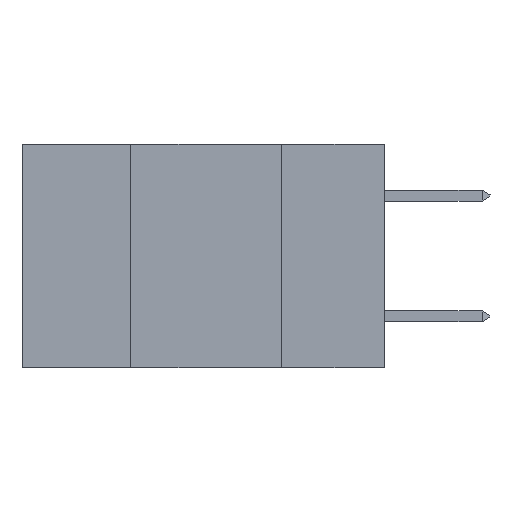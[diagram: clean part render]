
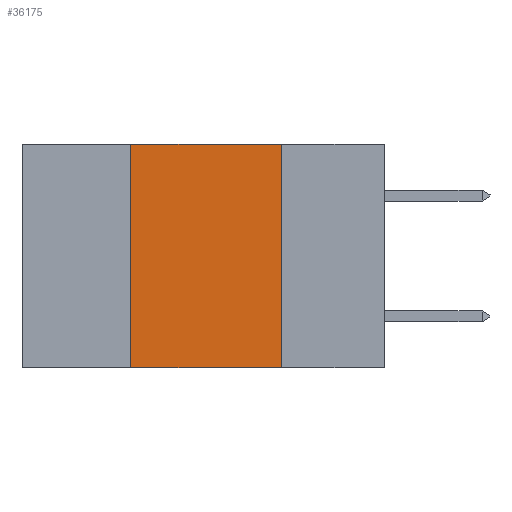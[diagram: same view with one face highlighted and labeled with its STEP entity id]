
A CAD part, left-side view. The second image highlights one B-rep face of the part: STEP entity #36175.
In plain terms, the highlighted planar face has unit normal (-1, 0, 0).
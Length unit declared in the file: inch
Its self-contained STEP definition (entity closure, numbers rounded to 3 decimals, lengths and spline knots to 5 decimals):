
#539 = CARTESIAN_POINT ( 'NONE',  ( 0., 0.42, -0.37 ) ) ;
#856 = LINE ( 'NONE', #30752, #36170 ) ;
#1742 = VERTEX_POINT ( 'NONE', #13037 ) ;
#3642 = DIRECTION ( 'NONE',  ( 1., 0., 0. ) ) ;
#7073 = EDGE_CURVE ( 'NONE', #12372, #36639, #12736, .T. ) ;
#8985 = EDGE_CURVE ( 'NONE', #12372, #1742, #856, .T. ) ;
#9290 = CARTESIAN_POINT ( 'NONE',  ( 0., 0.17, -0.37 ) ) ;
#10053 = CARTESIAN_POINT ( 'NONE',  ( 0., 0.6, -0.37 ) ) ;
#10506 = DIRECTION ( 'NONE',  ( 0., -1., 0. ) ) ;
#11003 = AXIS2_PLACEMENT_3D ( 'NONE', #36246, #3642, #24467 ) ;
#11580 = VECTOR ( 'NONE', #10506, 39.37008 ) ;
#12372 = VERTEX_POINT ( 'NONE', #539 ) ;
#12736 = LINE ( 'NONE', #10053, #35519 ) ;
#13037 = CARTESIAN_POINT ( 'NONE',  ( 0., 0.42, 0. ) ) ;
#13615 = LINE ( 'NONE', #23786, #21593 ) ;
#17338 = DIRECTION ( 'NONE',  ( 0., -1., 0. ) ) ;
#18328 = DIRECTION ( 'NONE',  ( 0., 0., 1. ) ) ;
#20653 = VERTEX_POINT ( 'NONE', #34096 ) ;
#21593 = VECTOR ( 'NONE', #29396, 39.37008 ) ;
#21905 = CARTESIAN_POINT ( 'NONE',  ( 0., 0.6, 0. ) ) ;
#23786 = CARTESIAN_POINT ( 'NONE',  ( 0., 0.17, 0. ) ) ;
#24299 = EDGE_CURVE ( 'NONE', #20653, #36639, #13615, .T. ) ;
#24467 = DIRECTION ( 'NONE',  ( 0., 0., -1. ) ) ;
#29249 = ORIENTED_EDGE ( 'NONE', *, *, #7073, .T. ) ;
#29396 = DIRECTION ( 'NONE',  ( 0., 0., -1. ) ) ;
#30752 = CARTESIAN_POINT ( 'NONE',  ( 0., 0.42, 0. ) ) ;
#30857 = ORIENTED_EDGE ( 'NONE', *, *, #31986, .F. ) ;
#31986 = EDGE_CURVE ( 'NONE', #1742, #20653, #36221, .T. ) ;
#33025 = PLANE ( 'NONE',  #11003 ) ;
#33587 = FACE_OUTER_BOUND ( 'NONE', #36972, .T. ) ;
#34096 = CARTESIAN_POINT ( 'NONE',  ( 0., 0.17, 0. ) ) ;
#34253 = ORIENTED_EDGE ( 'NONE', *, *, #8985, .F. ) ;
#34687 = ORIENTED_EDGE ( 'NONE', *, *, #24299, .F. ) ;
#35519 = VECTOR ( 'NONE', #17338, 39.37008 ) ;
#36170 = VECTOR ( 'NONE', #18328, 39.37008 ) ;
#36175 = ADVANCED_FACE ( 'NONE', ( #33587 ), #33025, .F. ) ;
#36221 = LINE ( 'NONE', #21905, #11580 ) ;
#36246 = CARTESIAN_POINT ( 'NONE',  ( 0., 0.6, 0. ) ) ;
#36639 = VERTEX_POINT ( 'NONE', #9290 ) ;
#36972 = EDGE_LOOP ( 'NONE', ( #34687, #30857, #34253, #29249 ) ) ;
